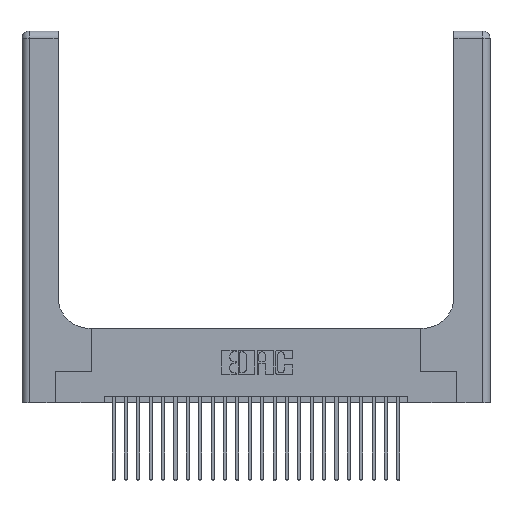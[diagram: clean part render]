
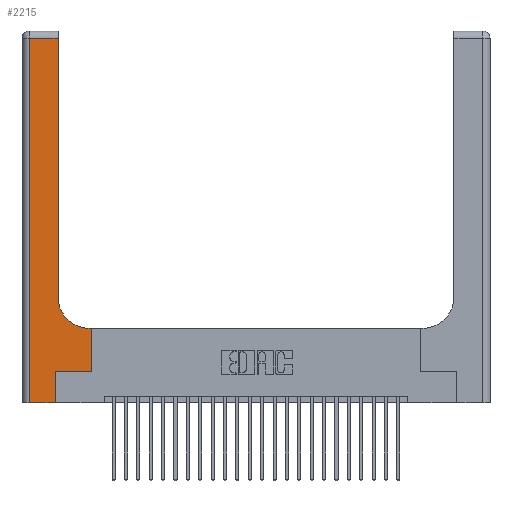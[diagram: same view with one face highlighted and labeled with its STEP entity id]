
A CAD part, top view. The second image highlights one B-rep face of the part: STEP entity #2215.
In plain terms, the highlighted planar face has unit normal (0, 0, 1).
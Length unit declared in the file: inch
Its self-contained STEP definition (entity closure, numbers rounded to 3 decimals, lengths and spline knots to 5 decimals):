
#123 = ORIENTED_EDGE ( 'NONE', *, *, #16731, .T. ) ;
#412 = LINE ( 'NONE', #21314, #26310 ) ;
#1443 = ORIENTED_EDGE ( 'NONE', *, *, #19185, .T. ) ;
#1515 = CARTESIAN_POINT ( 'NONE',  ( 0., 3., 0.37 ) ) ;
#1521 = ORIENTED_EDGE ( 'NONE', *, *, #5482, .T. ) ;
#1847 = VERTEX_POINT ( 'NONE', #15451 ) ;
#2091 = DIRECTION ( 'NONE',  ( -1., 0., 0. ) ) ;
#2188 = CARTESIAN_POINT ( 'NONE',  ( 0.269, 0.25, 0.37 ) ) ;
#2215 = ADVANCED_FACE ( 'NONE', ( #4360 ), #16012, .F. ) ;
#2950 = CARTESIAN_POINT ( 'NONE',  ( 0.269, 0., 0.37 ) ) ;
#3526 = EDGE_CURVE ( 'NONE', #4539, #1847, #12191, .T. ) ;
#4267 = VECTOR ( 'NONE', #9727, 39.37008 ) ;
#4360 = FACE_OUTER_BOUND ( 'NONE', #5819, .T. ) ;
#4539 = VERTEX_POINT ( 'NONE', #25746 ) ;
#5482 = EDGE_CURVE ( 'NONE', #20245, #19814, #9922, .T. ) ;
#5761 = VERTEX_POINT ( 'NONE', #18675 ) ;
#5819 = EDGE_LOOP ( 'NONE', ( #8485, #8565, #12678, #6273, #14989, #1521, #1443, #123, #7088 ) ) ;
#6273 = ORIENTED_EDGE ( 'NONE', *, *, #18058, .T. ) ;
#6683 = DIRECTION ( 'NONE',  ( 0., 1., 0. ) ) ;
#6934 = EDGE_CURVE ( 'NONE', #9735, #5761, #18967, .T. ) ;
#7088 = ORIENTED_EDGE ( 'NONE', *, *, #3526, .T. ) ;
#7902 = LINE ( 'NONE', #18802, #18067 ) ;
#8339 = VERTEX_POINT ( 'NONE', #21365 ) ;
#8485 = ORIENTED_EDGE ( 'NONE', *, *, #25450, .T. ) ;
#8565 = ORIENTED_EDGE ( 'NONE', *, *, #6934, .T. ) ;
#8605 = CARTESIAN_POINT ( 'NONE',  ( 0.5415, 0.85, 0.37 ) ) ;
#8998 = LINE ( 'NONE', #12528, #13779 ) ;
#9104 = LINE ( 'NONE', #14067, #19823 ) ;
#9635 = CARTESIAN_POINT ( 'NONE',  ( 0.2915, 2.94, 0.37 ) ) ;
#9727 = DIRECTION ( 'NONE',  ( 1., 0., 0. ) ) ;
#9735 = VERTEX_POINT ( 'NONE', #9635 ) ;
#9922 = LINE ( 'NONE', #25812, #4267 ) ;
#10704 = DIRECTION ( 'NONE',  ( 1., 0., 0. ) ) ;
#12078 = DIRECTION ( 'NONE',  ( -1., 0., 0. ) ) ;
#12134 = VECTOR ( 'NONE', #18958, 39.37008 ) ;
#12191 = CIRCLE ( 'NONE', #25123, 0.25 ) ;
#12528 = CARTESIAN_POINT ( 'NONE',  ( 0.2915, 0.6, 0.37 ) ) ;
#12678 = ORIENTED_EDGE ( 'NONE', *, *, #13325, .T. ) ;
#13325 = EDGE_CURVE ( 'NONE', #5761, #8339, #412, .T. ) ;
#13779 = VECTOR ( 'NONE', #2091, 39.37008 ) ;
#14067 = CARTESIAN_POINT ( 'NONE',  ( 0.269, 0., 0.37 ) ) ;
#14337 = DIRECTION ( 'NONE',  ( 0., 1., 0. ) ) ;
#14361 = DIRECTION ( 'NONE',  ( -1., 0., 0. ) ) ;
#14367 = VERTEX_POINT ( 'NONE', #2950 ) ;
#14601 = AXIS2_PLACEMENT_3D ( 'NONE', #1515, #24049, #12078 ) ;
#14989 = ORIENTED_EDGE ( 'NONE', *, *, #25341, .T. ) ;
#15451 = CARTESIAN_POINT ( 'NONE',  ( 0.2915, 0.85, 0.37 ) ) ;
#16012 = PLANE ( 'NONE',  #14601 ) ;
#16731 = EDGE_CURVE ( 'NONE', #26231, #4539, #8998, .T. ) ;
#17317 = CARTESIAN_POINT ( 'NONE',  ( 0.5585, 0.6, 0.37 ) ) ;
#17931 = VECTOR ( 'NONE', #6683, 39.37008 ) ;
#18058 = EDGE_CURVE ( 'NONE', #8339, #14367, #22796, .T. ) ;
#18067 = VECTOR ( 'NONE', #24723, 39.37008 ) ;
#18675 = CARTESIAN_POINT ( 'NONE',  ( 0.06, 2.94, 0.37 ) ) ;
#18802 = CARTESIAN_POINT ( 'NONE',  ( 0.5585, 0.25, 0.37 ) ) ;
#18868 = CARTESIAN_POINT ( 'NONE',  ( 0.5585, 0.25, 0.37 ) ) ;
#18958 = DIRECTION ( 'NONE',  ( 1., 0., 0. ) ) ;
#18967 = LINE ( 'NONE', #24282, #22413 ) ;
#19185 = EDGE_CURVE ( 'NONE', #19814, #26231, #7902, .T. ) ;
#19814 = VERTEX_POINT ( 'NONE', #18868 ) ;
#19823 = VECTOR ( 'NONE', #14337, 39.37008 ) ;
#20245 = VERTEX_POINT ( 'NONE', #2188 ) ;
#21314 = CARTESIAN_POINT ( 'NONE',  ( 0.06, 3., 0.37 ) ) ;
#21365 = CARTESIAN_POINT ( 'NONE',  ( 0.06, 0., 0.37 ) ) ;
#22413 = VECTOR ( 'NONE', #14361, 39.37008 ) ;
#22643 = LINE ( 'NONE', #24871, #17931 ) ;
#22705 = DIRECTION ( 'NONE',  ( 0., 0., -1. ) ) ;
#22796 = LINE ( 'NONE', #24878, #12134 ) ;
#23323 = DIRECTION ( 'NONE',  ( 0., -1., 0. ) ) ;
#24049 = DIRECTION ( 'NONE',  ( 0., 0., -1. ) ) ;
#24282 = CARTESIAN_POINT ( 'NONE',  ( 0., 2.94, 0.37 ) ) ;
#24723 = DIRECTION ( 'NONE',  ( 0., 1., 0. ) ) ;
#24871 = CARTESIAN_POINT ( 'NONE',  ( 0.2915, 3., 0.37 ) ) ;
#24878 = CARTESIAN_POINT ( 'NONE',  ( 0., 0., 0.37 ) ) ;
#25123 = AXIS2_PLACEMENT_3D ( 'NONE', #8605, #22705, #10704 ) ;
#25341 = EDGE_CURVE ( 'NONE', #14367, #20245, #9104, .T. ) ;
#25450 = EDGE_CURVE ( 'NONE', #1847, #9735, #22643, .T. ) ;
#25746 = CARTESIAN_POINT ( 'NONE',  ( 0.5415, 0.6, 0.37 ) ) ;
#25812 = CARTESIAN_POINT ( 'NONE',  ( 0.269, 0.25, 0.37 ) ) ;
#26231 = VERTEX_POINT ( 'NONE', #17317 ) ;
#26310 = VECTOR ( 'NONE', #23323, 39.37008 ) ;
